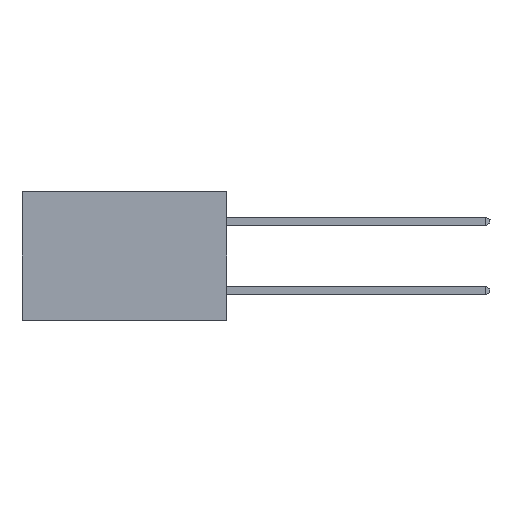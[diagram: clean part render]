
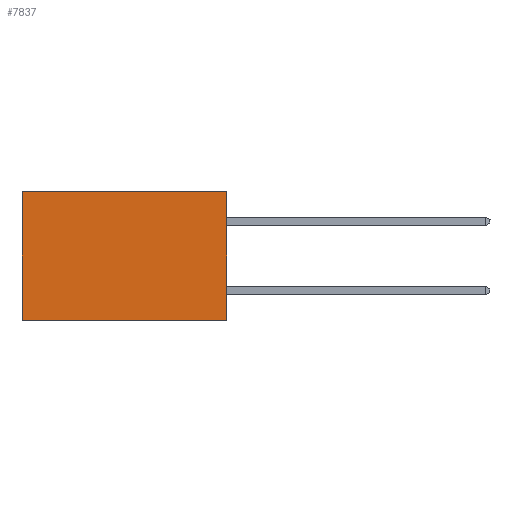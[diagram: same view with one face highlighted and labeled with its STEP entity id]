
A CAD part, left-side view. The second image highlights one B-rep face of the part: STEP entity #7837.
In plain terms, the highlighted planar face has unit normal (-1, 0, 0).
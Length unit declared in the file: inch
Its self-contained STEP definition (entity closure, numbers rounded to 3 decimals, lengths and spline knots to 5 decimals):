
#1389 = FACE_OUTER_BOUND ( 'NONE', #11434, .T. ) ;
#1896 = DIRECTION ( 'NONE',  ( 0., 0., -1. ) ) ;
#1959 = ORIENTED_EDGE ( 'NONE', *, *, #2433, .F. ) ;
#2160 = EDGE_CURVE ( 'NONE', #14493, #11361, #11740, .T. ) ;
#2312 = CARTESIAN_POINT ( 'NONE',  ( 0.277, 0., -0.37 ) ) ;
#2433 = EDGE_CURVE ( 'NONE', #11361, #14589, #4406, .T. ) ;
#3069 = EDGE_CURVE ( 'NONE', #13387, #14589, #5745, .T. ) ;
#3279 = CARTESIAN_POINT ( 'NONE',  ( 0.277, 0., 0. ) ) ;
#3519 = DIRECTION ( 'NONE',  ( 0., 1., 0. ) ) ;
#4336 = DIRECTION ( 'NONE',  ( 0., 0., -1. ) ) ;
#4406 = LINE ( 'NONE', #11978, #14142 ) ;
#4989 = VECTOR ( 'NONE', #1896, 39.37008 ) ;
#5349 = VECTOR ( 'NONE', #4336, 39.37008 ) ;
#5745 = LINE ( 'NONE', #12861, #5349 ) ;
#5758 = ORIENTED_EDGE ( 'NONE', *, *, #10092, .T. ) ;
#6708 = ORIENTED_EDGE ( 'NONE', *, *, #3069, .T. ) ;
#6735 = CARTESIAN_POINT ( 'NONE',  ( 0.277, 0.59, 0. ) ) ;
#7837 = ADVANCED_FACE ( 'NONE', ( #1389 ), #10174, .F. ) ;
#8679 = ORIENTED_EDGE ( 'NONE', *, *, #2160, .F. ) ;
#9981 = DIRECTION ( 'NONE',  ( 0., 0., -1. ) ) ;
#10007 = DIRECTION ( 'NONE',  ( 1., 0., 0. ) ) ;
#10082 = CARTESIAN_POINT ( 'NONE',  ( 0.277, 0., -0.37 ) ) ;
#10092 = EDGE_CURVE ( 'NONE', #14493, #13387, #12477, .T. ) ;
#10174 = PLANE ( 'NONE',  #16153 ) ;
#10407 = CARTESIAN_POINT ( 'NONE',  ( 0.277, 0.59, -0.37 ) ) ;
#11361 = VERTEX_POINT ( 'NONE', #13422 ) ;
#11434 = EDGE_LOOP ( 'NONE', ( #6708, #1959, #8679, #5758 ) ) ;
#11740 = LINE ( 'NONE', #2312, #4989 ) ;
#11978 = CARTESIAN_POINT ( 'NONE',  ( 0.277, 0., -0.37 ) ) ;
#12057 = DIRECTION ( 'NONE',  ( 0., 1., 0. ) ) ;
#12477 = LINE ( 'NONE', #3279, #15401 ) ;
#12756 = CARTESIAN_POINT ( 'NONE',  ( 0.277, 0., 0. ) ) ;
#12861 = CARTESIAN_POINT ( 'NONE',  ( 0.277, 0.59, -0.37 ) ) ;
#13387 = VERTEX_POINT ( 'NONE', #6735 ) ;
#13422 = CARTESIAN_POINT ( 'NONE',  ( 0.277, 0., -0.37 ) ) ;
#14142 = VECTOR ( 'NONE', #12057, 39.37008 ) ;
#14493 = VERTEX_POINT ( 'NONE', #12756 ) ;
#14589 = VERTEX_POINT ( 'NONE', #10407 ) ;
#15401 = VECTOR ( 'NONE', #3519, 39.37008 ) ;
#16153 = AXIS2_PLACEMENT_3D ( 'NONE', #10082, #10007, #9981 ) ;
